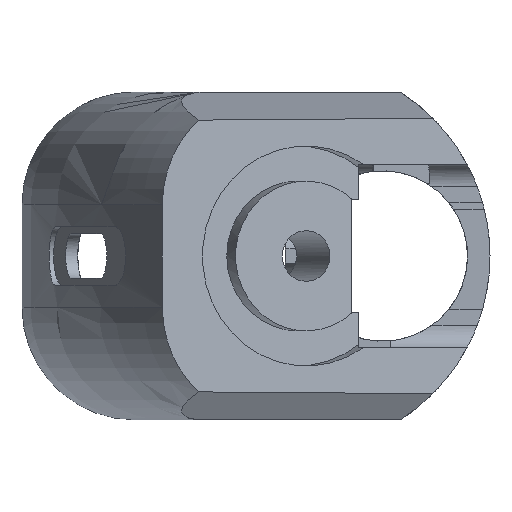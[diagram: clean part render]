
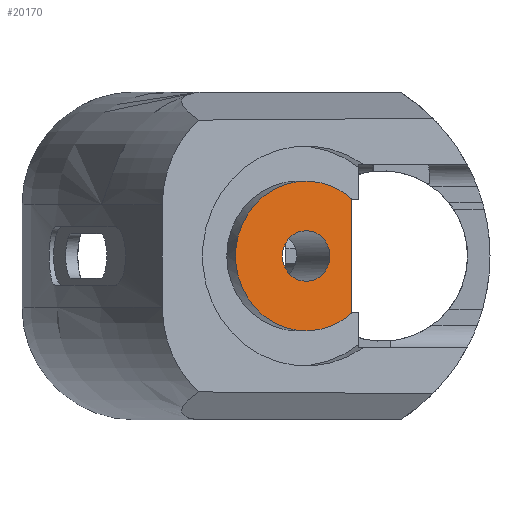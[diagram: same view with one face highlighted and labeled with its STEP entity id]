
A CAD part, left-side view. The second image highlights one B-rep face of the part: STEP entity #20170.
In plain terms, the highlighted planar face has unit normal (-0.943, -0.334, 0).
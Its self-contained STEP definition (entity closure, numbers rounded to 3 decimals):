
#4301 = PLANE('',#4302);
#4302 = AXIS2_PLACEMENT_3D('',#4303,#4304,#4305);
#4303 = CARTESIAN_POINT('',(-152.4,18.796,7.62));
#4304 = DIRECTION('',(0.,-1.,0.));
#4305 = DIRECTION('',(0.,0.,-1.));
#4350 = CYLINDRICAL_SURFACE('',#4351,3.429);
#4351 = AXIS2_PLACEMENT_3D('',#4352,#4353,#4354);
#4352 = CARTESIAN_POINT('',(-202.64,24.947,0.));
#4353 = DIRECTION('',(-0.943,-0.334,0.));
#4354 = DIRECTION('',(0.334,-0.943,0.));
#11928 = CYLINDRICAL_SURFACE('',#11929,10.16);
#11929 = AXIS2_PLACEMENT_3D('',#11930,#11931,#11932);
#11930 = CARTESIAN_POINT('',(-202.64,24.947,0.)
  );
#11931 = DIRECTION('',(-0.943,-0.334,0.));
#11932 = DIRECTION('',(0.334,-0.943,0.));
#12061 = VERTEX_POINT('',#12062);
#12062 = CARTESIAN_POINT('',(-200.461,18.796,7.62));
#12076 = PLANE('',#12077);
#12077 = AXIS2_PLACEMENT_3D('',#12078,#12079,#12080);
#12078 = CARTESIAN_POINT('',(-152.4,17.78,7.62));
#12079 = DIRECTION('',(0.,0.,-1.));
#12080 = DIRECTION('',(0.,1.,0.));
#12088 = EDGE_CURVE('',#12061,#12089,#12091,.T.);
#12089 = VERTEX_POINT('',#12090);
#12090 = CARTESIAN_POINT('',(-200.461,18.796,-7.62));
#12091 = SURFACE_CURVE('',#12092,(#12096,#12102),.PCURVE_S1.);
#12092 = LINE('',#12093,#12094);
#12093 = CARTESIAN_POINT('',(-200.461,18.796,-7.303));
#12094 = VECTOR('',#12095,1.);
#12095 = DIRECTION('',(0.,0.,-1.));
#12096 = PCURVE('',#4301,#12097);
#12097 = DEFINITIONAL_REPRESENTATION('',(#12098),#12101);
#12098 = B_SPLINE_CURVE_WITH_KNOTS('',1,(#12099,#12100),.UNSPECIFIED.,
  .F.,.F.,(2,2),(-14.923,0.318),.PIECEWISE_BEZIER_KNOTS.);
#12099 = CARTESIAN_POINT('',(0.,-48.061));
#12100 = CARTESIAN_POINT('',(15.24,-48.061));
#12101 = ( GEOMETRIC_REPRESENTATION_CONTEXT(2) 
PARAMETRIC_REPRESENTATION_CONTEXT() REPRESENTATION_CONTEXT('2D SPACE',''
  ) );
#12102 = PCURVE('',#12103,#12108);
#12103 = PLANE('',#12104);
#12104 = AXIS2_PLACEMENT_3D('',#12105,#12106,#12107);
#12105 = CARTESIAN_POINT('',(-209.55,44.45,-22.225));
#12106 = DIRECTION('',(0.943,0.334,0.));
#12107 = DIRECTION('',(0.334,-0.943,0.));
#12108 = DEFINITIONAL_REPRESENTATION('',(#12109),#12112);
#12109 = B_SPLINE_CURVE_WITH_KNOTS('',1,(#12110,#12111),.UNSPECIFIED.,
  .F.,.F.,(2,2),(-14.923,0.318),.PIECEWISE_BEZIER_KNOTS.);
#12110 = CARTESIAN_POINT('',(27.216,-29.845));
#12111 = CARTESIAN_POINT('',(27.216,-14.605));
#12112 = ( GEOMETRIC_REPRESENTATION_CONTEXT(2) 
PARAMETRIC_REPRESENTATION_CONTEXT() REPRESENTATION_CONTEXT('2D SPACE',''
  ) );
#12130 = PLANE('',#12131);
#12131 = AXIS2_PLACEMENT_3D('',#12132,#12133,#12134);
#12132 = CARTESIAN_POINT('',(-152.4,18.796,-7.62));
#12133 = DIRECTION('',(0.,0.,1.));
#12134 = DIRECTION('',(0.,-1.,0.));
#12228 = EDGE_CURVE('',#12229,#12229,#12231,.T.);
#12229 = VERTEX_POINT('',#12230);
#12230 = CARTESIAN_POINT('',(-201.495,21.715,0.
    ));
#12231 = SURFACE_CURVE('',#12232,(#12237,#12244),.PCURVE_S1.);
#12232 = CIRCLE('',#12233,3.429);
#12233 = AXIS2_PLACEMENT_3D('',#12234,#12235,#12236);
#12234 = CARTESIAN_POINT('',(-202.64,24.947,0.)
  );
#12235 = DIRECTION('',(-0.943,-0.334,
    0.));
#12236 = DIRECTION('',(0.334,-0.943,0.));
#12237 = PCURVE('',#4350,#12238);
#12238 = DEFINITIONAL_REPRESENTATION('',(#12239),#12243);
#12239 = LINE('',#12240,#12241);
#12240 = CARTESIAN_POINT('',(0.,0.));
#12241 = VECTOR('',#12242,1.);
#12242 = DIRECTION('',(1.,0.));
#12243 = ( GEOMETRIC_REPRESENTATION_CONTEXT(2) 
PARAMETRIC_REPRESENTATION_CONTEXT() REPRESENTATION_CONTEXT('2D SPACE',''
  ) );
#12244 = PCURVE('',#12103,#12245);
#12245 = DEFINITIONAL_REPRESENTATION('',(#12246),#12254);
#12246 = ( BOUNDED_CURVE() B_SPLINE_CURVE(2,(#12247,#12248,#12249,#12250
    ,#12251,#12252,#12253),.UNSPECIFIED.,.T.,.F.) 
B_SPLINE_CURVE_WITH_KNOTS((1,2,2,2,2,1),(-2.094,0.,
    2.094,4.189,6.283,8.378),
.UNSPECIFIED.) CURVE() GEOMETRIC_REPRESENTATION_ITEM() 
RATIONAL_B_SPLINE_CURVE((1.,0.5,1.,0.5,1.,0.5,1.)) REPRESENTATION_ITEM(
  '') );
#12247 = CARTESIAN_POINT('',(24.12,-22.225));
#12248 = CARTESIAN_POINT('',(24.12,-28.164));
#12249 = CARTESIAN_POINT('',(18.976,-25.195));
#12250 = CARTESIAN_POINT('',(13.833,-22.225));
#12251 = CARTESIAN_POINT('',(18.976,-19.255));
#12252 = CARTESIAN_POINT('',(24.12,-16.286));
#12253 = CARTESIAN_POINT('',(24.12,-22.225));
#12254 = ( GEOMETRIC_REPRESENTATION_CONTEXT(2) 
PARAMETRIC_REPRESENTATION_CONTEXT() REPRESENTATION_CONTEXT('2D SPACE',''
  ) );
#20076 = EDGE_CURVE('',#20077,#20079,#20081,.T.);
#20077 = VERTEX_POINT('',#20078);
#20078 = CARTESIAN_POINT('',(-200.396,18.613,7.62));
#20079 = VERTEX_POINT('',#20080);
#20080 = CARTESIAN_POINT('',(-200.396,18.613,-7.62));
#20081 = SURFACE_CURVE('',#20082,(#20087,#20094),.PCURVE_S1.);
#20082 = CIRCLE('',#20083,10.16);
#20083 = AXIS2_PLACEMENT_3D('',#20084,#20085,#20086);
#20084 = CARTESIAN_POINT('',(-202.64,24.947,0.)
  );
#20085 = DIRECTION('',(-0.943,-0.334,
    0.));
#20086 = DIRECTION('',(0.334,-0.943,0.));
#20087 = PCURVE('',#11928,#20088);
#20088 = DEFINITIONAL_REPRESENTATION('',(#20089),#20093);
#20089 = LINE('',#20090,#20091);
#20090 = CARTESIAN_POINT('',(0.,0.));
#20091 = VECTOR('',#20092,1.);
#20092 = DIRECTION('',(1.,0.));
#20093 = ( GEOMETRIC_REPRESENTATION_CONTEXT(2) 
PARAMETRIC_REPRESENTATION_CONTEXT() REPRESENTATION_CONTEXT('2D SPACE',''
  ) );
#20094 = PCURVE('',#12103,#20095);
#20095 = DEFINITIONAL_REPRESENTATION('',(#20096),#20104);
#20096 = ( BOUNDED_CURVE() B_SPLINE_CURVE(2,(#20097,#20098,#20099,#20100
    ,#20101,#20102,#20103),.UNSPECIFIED.,.T.,.F.) 
B_SPLINE_CURVE_WITH_KNOTS((1,2,2,2,2,1),(-2.094,0.,
    2.094,4.189,6.283,8.378),
.UNSPECIFIED.) CURVE() GEOMETRIC_REPRESENTATION_ITEM() 
RATIONAL_B_SPLINE_CURVE((1.,0.5,1.,0.5,1.,0.5,1.)) REPRESENTATION_ITEM(
  '') );
#20097 = CARTESIAN_POINT('',(30.851,-22.225));
#20098 = CARTESIAN_POINT('',(30.851,-39.823));
#20099 = CARTESIAN_POINT('',(15.611,-31.024));
#20100 = CARTESIAN_POINT('',(0.371,-22.225));
#20101 = CARTESIAN_POINT('',(15.611,-13.426));
#20102 = CARTESIAN_POINT('',(30.851,-4.627));
#20103 = CARTESIAN_POINT('',(30.851,-22.225));
#20104 = ( GEOMETRIC_REPRESENTATION_CONTEXT(2) 
PARAMETRIC_REPRESENTATION_CONTEXT() REPRESENTATION_CONTEXT('2D SPACE',''
  ) );
#20152 = EDGE_CURVE('',#12089,#20079,#20153,.T.);
#20153 = SURFACE_CURVE('',#20154,(#20158,#20164),.PCURVE_S1.);
#20154 = LINE('',#20155,#20156);
#20155 = CARTESIAN_POINT('',(-202.326,24.059,-7.62));
#20156 = VECTOR('',#20157,1.);
#20157 = DIRECTION('',(0.334,-0.943,0.));
#20158 = PCURVE('',#12130,#20159);
#20159 = DEFINITIONAL_REPRESENTATION('',(#20160),#20163);
#20160 = B_SPLINE_CURVE_WITH_KNOTS('',1,(#20161,#20162),.UNSPECIFIED.,
  .F.,.F.,(2,2),(5.583,6.661),
  .PIECEWISE_BEZIER_KNOTS.);
#20161 = CARTESIAN_POINT('',(0.,-48.061));
#20162 = CARTESIAN_POINT('',(1.016,-47.701));
#20163 = ( GEOMETRIC_REPRESENTATION_CONTEXT(2) 
PARAMETRIC_REPRESENTATION_CONTEXT() REPRESENTATION_CONTEXT('2D SPACE',''
  ) );
#20164 = PCURVE('',#12103,#20165);
#20165 = DEFINITIONAL_REPRESENTATION('',(#20166),#20169);
#20166 = B_SPLINE_CURVE_WITH_KNOTS('',1,(#20167,#20168),.UNSPECIFIED.,
  .F.,.F.,(2,2),(5.583,6.661),
  .PIECEWISE_BEZIER_KNOTS.);
#20167 = CARTESIAN_POINT('',(27.216,-14.605));
#20168 = CARTESIAN_POINT('',(28.294,-14.605));
#20169 = ( GEOMETRIC_REPRESENTATION_CONTEXT(2) 
PARAMETRIC_REPRESENTATION_CONTEXT() REPRESENTATION_CONTEXT('2D SPACE',''
  ) );
#20170 = ADVANCED_FACE('',(#20171,#20195),#12103,.F.);
#20171 = FACE_BOUND('',#20172,.F.);
#20172 = EDGE_LOOP('',(#20173,#20174,#20175,#20194));
#20173 = ORIENTED_EDGE('',*,*,#20152,.T.);
#20174 = ORIENTED_EDGE('',*,*,#20076,.F.);
#20175 = ORIENTED_EDGE('',*,*,#20176,.T.);
#20176 = EDGE_CURVE('',#20077,#12061,#20177,.T.);
#20177 = SURFACE_CURVE('',#20178,(#20182,#20188),.PCURVE_S1.);
#20178 = LINE('',#20179,#20180);
#20179 = CARTESIAN_POINT('',(-202.166,23.607,7.62));
#20180 = VECTOR('',#20181,1.);
#20181 = DIRECTION('',(-0.334,0.943,0.));
#20182 = PCURVE('',#12103,#20183);
#20183 = DEFINITIONAL_REPRESENTATION('',(#20184),#20187);
#20184 = B_SPLINE_CURVE_WITH_KNOTS('',1,(#20185,#20186),.UNSPECIFIED.,
  .F.,.F.,(2,2),(-6.182,-5.104),
  .PIECEWISE_BEZIER_KNOTS.);
#20185 = CARTESIAN_POINT('',(28.294,-29.845));
#20186 = CARTESIAN_POINT('',(27.216,-29.845));
#20187 = ( GEOMETRIC_REPRESENTATION_CONTEXT(2) 
PARAMETRIC_REPRESENTATION_CONTEXT() REPRESENTATION_CONTEXT('2D SPACE',''
  ) );
#20188 = PCURVE('',#12076,#20189);
#20189 = DEFINITIONAL_REPRESENTATION('',(#20190),#20193);
#20190 = B_SPLINE_CURVE_WITH_KNOTS('',1,(#20191,#20192),.UNSPECIFIED.,
  .F.,.F.,(2,2),(-6.182,-5.104),
  .PIECEWISE_BEZIER_KNOTS.);
#20191 = CARTESIAN_POINT('',(0.,-47.701));
#20192 = CARTESIAN_POINT('',(1.016,-48.061));
#20193 = ( GEOMETRIC_REPRESENTATION_CONTEXT(2) 
PARAMETRIC_REPRESENTATION_CONTEXT() REPRESENTATION_CONTEXT('2D SPACE',''
  ) );
#20194 = ORIENTED_EDGE('',*,*,#12088,.T.);
#20195 = FACE_BOUND('',#20196,.F.);
#20196 = EDGE_LOOP('',(#20197));
#20197 = ORIENTED_EDGE('',*,*,#12228,.T.);
